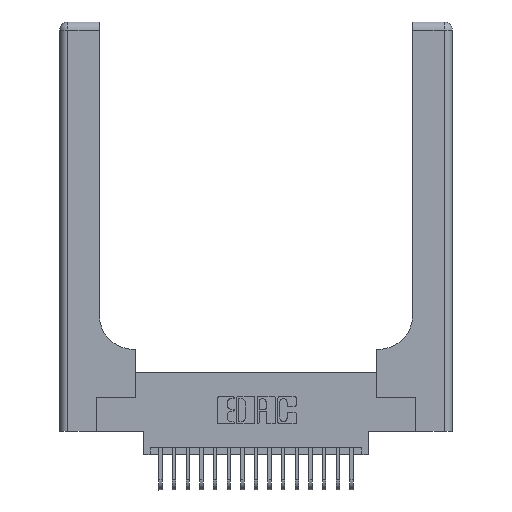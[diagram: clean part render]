
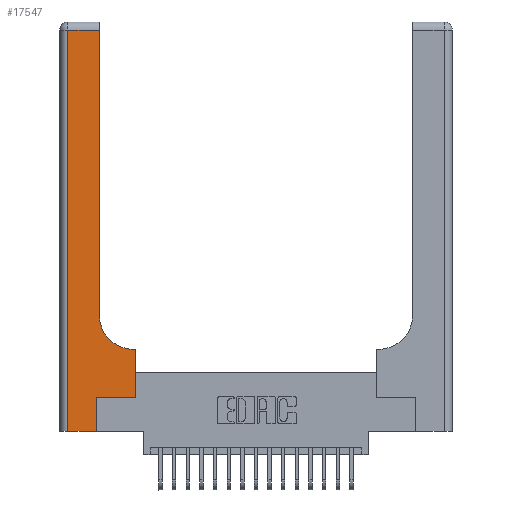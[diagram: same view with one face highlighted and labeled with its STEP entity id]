
A CAD part, top view. The second image highlights one B-rep face of the part: STEP entity #17547.
In plain terms, the highlighted planar face has unit normal (0, 0, 1).
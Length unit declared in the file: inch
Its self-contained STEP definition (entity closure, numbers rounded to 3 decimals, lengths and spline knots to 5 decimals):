
#567 = CARTESIAN_POINT ( 'NONE',  ( 0., 0., 0.37 ) ) ;
#922 = EDGE_CURVE ( 'NONE', #3497, #10258, #18898, .T. ) ;
#1162 = DIRECTION ( 'NONE',  ( -1., 0., 0. ) ) ;
#1418 = VERTEX_POINT ( 'NONE', #20152 ) ;
#1784 = CARTESIAN_POINT ( 'NONE',  ( 0.5585, 0.6, 0.37 ) ) ;
#2749 = VECTOR ( 'NONE', #3295, 39.37008 ) ;
#3295 = DIRECTION ( 'NONE',  ( 0., -1., 0. ) ) ;
#3331 = ORIENTED_EDGE ( 'NONE', *, *, #20071, .T. ) ;
#3405 = CARTESIAN_POINT ( 'NONE',  ( 0.06, 3., 0.37 ) ) ;
#3497 = VERTEX_POINT ( 'NONE', #3550 ) ;
#3550 = CARTESIAN_POINT ( 'NONE',  ( 0.06, 2.94, 0.37 ) ) ;
#3814 = CARTESIAN_POINT ( 'NONE',  ( 0.5415, 0.6, 0.37 ) ) ;
#4071 = DIRECTION ( 'NONE',  ( 1., 0., 0. ) ) ;
#4267 = VECTOR ( 'NONE', #10377, 39.37008 ) ;
#4352 = LINE ( 'NONE', #15023, #8090 ) ;
#4459 = VECTOR ( 'NONE', #1162, 39.37008 ) ;
#4551 = CARTESIAN_POINT ( 'NONE',  ( 0.5415, 0.85, 0.37 ) ) ;
#5054 = EDGE_CURVE ( 'NONE', #5861, #19351, #14658, .T. ) ;
#5861 = VERTEX_POINT ( 'NONE', #3814 ) ;
#5883 = CARTESIAN_POINT ( 'NONE',  ( 0., 2.94, 0.37 ) ) ;
#6128 = DIRECTION ( 'NONE',  ( 1., 0., 0. ) ) ;
#6538 = EDGE_CURVE ( 'NONE', #19351, #12580, #15785, .T. ) ;
#6900 = EDGE_CURVE ( 'NONE', #7720, #1418, #16753, .T. ) ;
#6998 = DIRECTION ( 'NONE',  ( 0., 0., -1. ) ) ;
#7181 = CARTESIAN_POINT ( 'NONE',  ( 0.269, 0., 0.37 ) ) ;
#7382 = VERTEX_POINT ( 'NONE', #1784 ) ;
#7564 = VECTOR ( 'NONE', #4071, 39.37008 ) ;
#7720 = VERTEX_POINT ( 'NONE', #7181 ) ;
#7937 = DIRECTION ( 'NONE',  ( -1., 0., 0. ) ) ;
#8090 = VECTOR ( 'NONE', #11940, 39.37008 ) ;
#8701 = ORIENTED_EDGE ( 'NONE', *, *, #6900, .T. ) ;
#8783 = CARTESIAN_POINT ( 'NONE',  ( 0.269, 0., 0.37 ) ) ;
#8812 = VECTOR ( 'NONE', #7937, 39.37008 ) ;
#8885 = DIRECTION ( 'NONE',  ( 0., 1., 0. ) ) ;
#9632 = ORIENTED_EDGE ( 'NONE', *, *, #6538, .T. ) ;
#9671 = AXIS2_PLACEMENT_3D ( 'NONE', #4551, #15500, #6128 ) ;
#10236 = ORIENTED_EDGE ( 'NONE', *, *, #922, .T. ) ;
#10258 = VERTEX_POINT ( 'NONE', #19409 ) ;
#10377 = DIRECTION ( 'NONE',  ( 0., 1., 0. ) ) ;
#10385 = VECTOR ( 'NONE', #11673, 39.37008 ) ;
#10437 = CARTESIAN_POINT ( 'NONE',  ( 0.5585, 0.25, 0.37 ) ) ;
#11005 = ORIENTED_EDGE ( 'NONE', *, *, #11978, .T. ) ;
#11028 = EDGE_CURVE ( 'NONE', #12580, #3497, #13320, .T. ) ;
#11055 = ORIENTED_EDGE ( 'NONE', *, *, #18908, .T. ) ;
#11617 = AXIS2_PLACEMENT_3D ( 'NONE', #13271, #6998, #17910 ) ;
#11673 = DIRECTION ( 'NONE',  ( 1., 0., 0. ) ) ;
#11940 = DIRECTION ( 'NONE',  ( 0., 1., 0. ) ) ;
#11978 = EDGE_CURVE ( 'NONE', #10258, #7720, #13988, .T. ) ;
#12027 = ORIENTED_EDGE ( 'NONE', *, *, #5054, .T. ) ;
#12199 = VECTOR ( 'NONE', #8885, 39.37008 ) ;
#12580 = VERTEX_POINT ( 'NONE', #12760 ) ;
#12760 = CARTESIAN_POINT ( 'NONE',  ( 0.2915, 2.94, 0.37 ) ) ;
#13271 = CARTESIAN_POINT ( 'NONE',  ( 0., 3., 0.37 ) ) ;
#13320 = LINE ( 'NONE', #5883, #4459 ) ;
#13546 = ORIENTED_EDGE ( 'NONE', *, *, #11028, .T. ) ;
#13819 = EDGE_CURVE ( 'NONE', #7382, #5861, #17033, .T. ) ;
#13988 = LINE ( 'NONE', #567, #10385 ) ;
#14658 = CIRCLE ( 'NONE', #9671, 0.25 ) ;
#14769 = ORIENTED_EDGE ( 'NONE', *, *, #13819, .T. ) ;
#15023 = CARTESIAN_POINT ( 'NONE',  ( 0.5585, 0.25, 0.37 ) ) ;
#15050 = CARTESIAN_POINT ( 'NONE',  ( 0.269, 0.25, 0.37 ) ) ;
#15500 = DIRECTION ( 'NONE',  ( 0., 0., -1. ) ) ;
#15665 = CARTESIAN_POINT ( 'NONE',  ( 0.2915, 0.6, 0.37 ) ) ;
#15785 = LINE ( 'NONE', #16593, #12199 ) ;
#15918 = FACE_OUTER_BOUND ( 'NONE', #19301, .T. ) ;
#16026 = VERTEX_POINT ( 'NONE', #10437 ) ;
#16334 = LINE ( 'NONE', #15050, #7564 ) ;
#16361 = PLANE ( 'NONE',  #11617 ) ;
#16593 = CARTESIAN_POINT ( 'NONE',  ( 0.2915, 3., 0.37 ) ) ;
#16753 = LINE ( 'NONE', #8783, #4267 ) ;
#17033 = LINE ( 'NONE', #15665, #8812 ) ;
#17547 = ADVANCED_FACE ( 'NONE', ( #15918 ), #16361, .F. ) ;
#17910 = DIRECTION ( 'NONE',  ( -1., 0., 0. ) ) ;
#18898 = LINE ( 'NONE', #3405, #2749 ) ;
#18908 = EDGE_CURVE ( 'NONE', #16026, #7382, #4352, .T. ) ;
#19264 = CARTESIAN_POINT ( 'NONE',  ( 0.2915, 0.85, 0.37 ) ) ;
#19301 = EDGE_LOOP ( 'NONE', ( #9632, #13546, #10236, #11005, #8701, #3331, #11055, #14769, #12027 ) ) ;
#19351 = VERTEX_POINT ( 'NONE', #19264 ) ;
#19409 = CARTESIAN_POINT ( 'NONE',  ( 0.06, 0., 0.37 ) ) ;
#20071 = EDGE_CURVE ( 'NONE', #1418, #16026, #16334, .T. ) ;
#20152 = CARTESIAN_POINT ( 'NONE',  ( 0.269, 0.25, 0.37 ) ) ;
